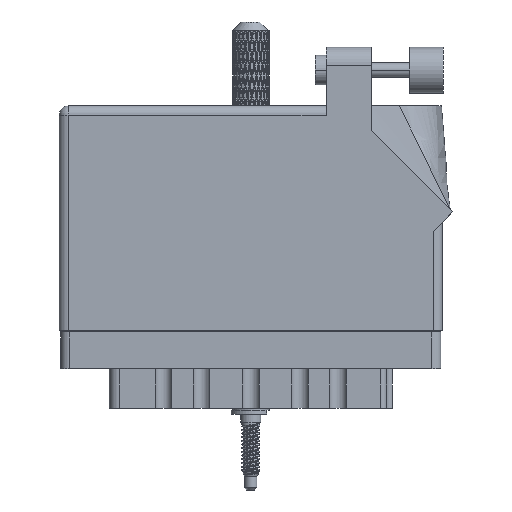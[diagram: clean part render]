
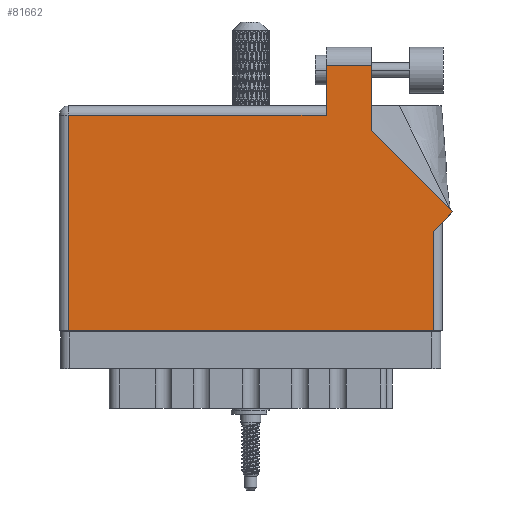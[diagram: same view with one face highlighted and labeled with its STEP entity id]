
A CAD part, front view. The second image highlights one B-rep face of the part: STEP entity #81662.
In plain terms, the highlighted face is planar.
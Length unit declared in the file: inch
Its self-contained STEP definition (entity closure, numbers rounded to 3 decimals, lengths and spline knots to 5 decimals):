
#2742 = EDGE_CURVE ( 'NONE', #32183, #31734, #59889, .T. ) ;
#4863 = DIRECTION ( 'NONE',  ( -1., 0., 0. ) ) ;
#5004 = VECTOR ( 'NONE', #4863, 39.37008 ) ;
#5295 = VERTEX_POINT ( 'NONE', #72208 ) ;
#5300 = ORIENTED_EDGE ( 'NONE', *, *, #14669, .T. ) ;
#5929 = DIRECTION ( 'NONE',  ( -0.707, 0.707, 0. ) ) ;
#6899 = EDGE_CURVE ( 'NONE', #31734, #95894, #73021, .T. ) ;
#7108 = ORIENTED_EDGE ( 'NONE', *, *, #30678, .T. ) ;
#7490 = CARTESIAN_POINT ( 'NONE',  ( 1.819, 1.53, 0. ) ) ;
#9343 = EDGE_CURVE ( 'NONE', #95894, #103327, #81716, .T. ) ;
#12216 = CARTESIAN_POINT ( 'NONE',  ( 2.126, 1.36442, 0. ) ) ;
#13255 = CARTESIAN_POINT ( 'NONE',  ( 2.55, 0.737, 0. ) ) ;
#13492 = ORIENTED_EDGE ( 'NONE', *, *, #16133, .T. ) ;
#13626 = DIRECTION ( 'NONE',  ( 0., 1., 0. ) ) ;
#14669 = EDGE_CURVE ( 'NONE', #82881, #86919, #70924, .T. ) ;
#16133 = EDGE_CURVE ( 'NONE', #22067, #108328, #16513, .T. ) ;
#16513 = LINE ( 'NONE', #100112, #69163 ) ;
#22067 = VERTEX_POINT ( 'NONE', #51374 ) ;
#23490 = VECTOR ( 'NONE', #80474, 39.37008 ) ;
#28532 = LINE ( 'NONE', #84219, #5004 ) ;
#29279 = CARTESIAN_POINT ( 'NONE',  ( 2.55, 0., 0. ) ) ;
#29332 = ORIENTED_EDGE ( 'NONE', *, *, #2742, .T. ) ;
#30678 = EDGE_CURVE ( 'NONE', #5295, #32183, #81972, .T. ) ;
#30780 = LINE ( 'NONE', #13255, #91743 ) ;
#31734 = VERTEX_POINT ( 'NONE', #48094 ) ;
#32183 = VERTEX_POINT ( 'NONE', #84432 ) ;
#33228 = DIRECTION ( 'NONE',  ( 0., 0., -1. ) ) ;
#34881 = VECTOR ( 'NONE', #88000, 39.37008 ) ;
#34944 = CARTESIAN_POINT ( 'NONE',  ( 0., 1.468, 0. ) ) ;
#35606 = CARTESIAN_POINT ( 'NONE',  ( 2.126, 1.36442, 0. ) ) ;
#37959 = FACE_OUTER_BOUND ( 'NONE', #58532, .T. ) ;
#44514 = VECTOR ( 'NONE', #65321, 39.37008 ) ;
#48094 = CARTESIAN_POINT ( 'NONE',  ( 0.062, 1.468, 0. ) ) ;
#51345 = DIRECTION ( 'NONE',  ( -1., 0., 0. ) ) ;
#51374 = CARTESIAN_POINT ( 'NONE',  ( 2.55, 0.675, 0. ) ) ;
#51649 = ORIENTED_EDGE ( 'NONE', *, *, #52848, .T. ) ;
#52848 = EDGE_CURVE ( 'NONE', #108328, #82881, #94462, .T. ) ;
#58532 = EDGE_LOOP ( 'NONE', ( #5300, #93854, #7108, #29332, #110427, #97787, #66408, #13492, #51649 ) ) ;
#58949 = CARTESIAN_POINT ( 'NONE',  ( 2.68271, 0.80771, 0. ) ) ;
#59889 = LINE ( 'NONE', #34944, #63946 ) ;
#62622 = CARTESIAN_POINT ( 'NONE',  ( 0., 0., 0. ) ) ;
#63946 = VECTOR ( 'NONE', #104625, 39.37008 ) ;
#65321 = DIRECTION ( 'NONE',  ( 0., 1., 0. ) ) ;
#66408 = ORIENTED_EDGE ( 'NONE', *, *, #84152, .T. ) ;
#69163 = VECTOR ( 'NONE', #73007, 39.37008 ) ;
#69710 = CARTESIAN_POINT ( 'NONE',  ( 0.062, 0., 0. ) ) ;
#70085 = DIRECTION ( 'NONE',  ( 0., -1., 0. ) ) ;
#70924 = LINE ( 'NONE', #35606, #44514 ) ;
#72208 = CARTESIAN_POINT ( 'NONE',  ( 1.819, 1.805, 0. ) ) ;
#73007 = DIRECTION ( 'NONE',  ( 0.707, 0.707, 0. ) ) ;
#73021 = LINE ( 'NONE', #69710, #82693 ) ;
#80474 = DIRECTION ( 'NONE',  ( 1., 0., 0. ) ) ;
#81662 = ADVANCED_FACE ( 'NONE', ( #37959 ), #104448, .F. ) ;
#81716 = LINE ( 'NONE', #62622, #23490 ) ;
#81972 = LINE ( 'NONE', #7490, #34881 ) ;
#82338 = CARTESIAN_POINT ( 'NONE',  ( 0.062, 0., 0. ) ) ;
#82693 = VECTOR ( 'NONE', #70085, 39.37008 ) ;
#82881 = VERTEX_POINT ( 'NONE', #12216 ) ;
#83447 = CARTESIAN_POINT ( 'NONE',  ( 2.68271, 0.80771, 0. ) ) ;
#84152 = EDGE_CURVE ( 'NONE', #103327, #22067, #30780, .T. ) ;
#84219 = CARTESIAN_POINT ( 'NONE',  ( 1.819, 1.805, 0. ) ) ;
#84432 = CARTESIAN_POINT ( 'NONE',  ( 1.819, 1.468, 0. ) ) ;
#86919 = VERTEX_POINT ( 'NONE', #89230 ) ;
#88000 = DIRECTION ( 'NONE',  ( 0., -1., 0. ) ) ;
#89230 = CARTESIAN_POINT ( 'NONE',  ( 2.126, 1.805, 0. ) ) ;
#91743 = VECTOR ( 'NONE', #13626, 39.37008 ) ;
#93854 = ORIENTED_EDGE ( 'NONE', *, *, #106231, .T. ) ;
#94462 = LINE ( 'NONE', #58949, #108320 ) ;
#95894 = VERTEX_POINT ( 'NONE', #82338 ) ;
#97787 = ORIENTED_EDGE ( 'NONE', *, *, #9343, .T. ) ;
#98285 = AXIS2_PLACEMENT_3D ( 'NONE', #113798, #33228, #51345 ) ;
#100112 = CARTESIAN_POINT ( 'NONE',  ( 2.612, 0.737, 0. ) ) ;
#103327 = VERTEX_POINT ( 'NONE', #29279 ) ;
#104448 = PLANE ( 'NONE',  #98285 ) ;
#104625 = DIRECTION ( 'NONE',  ( -1., 0., 0. ) ) ;
#106231 = EDGE_CURVE ( 'NONE', #86919, #5295, #28532, .T. ) ;
#108320 = VECTOR ( 'NONE', #5929, 39.37008 ) ;
#108328 = VERTEX_POINT ( 'NONE', #83447 ) ;
#110427 = ORIENTED_EDGE ( 'NONE', *, *, #6899, .T. ) ;
#113798 = CARTESIAN_POINT ( 'NONE',  ( 0., 1.53, 0. ) ) ;
